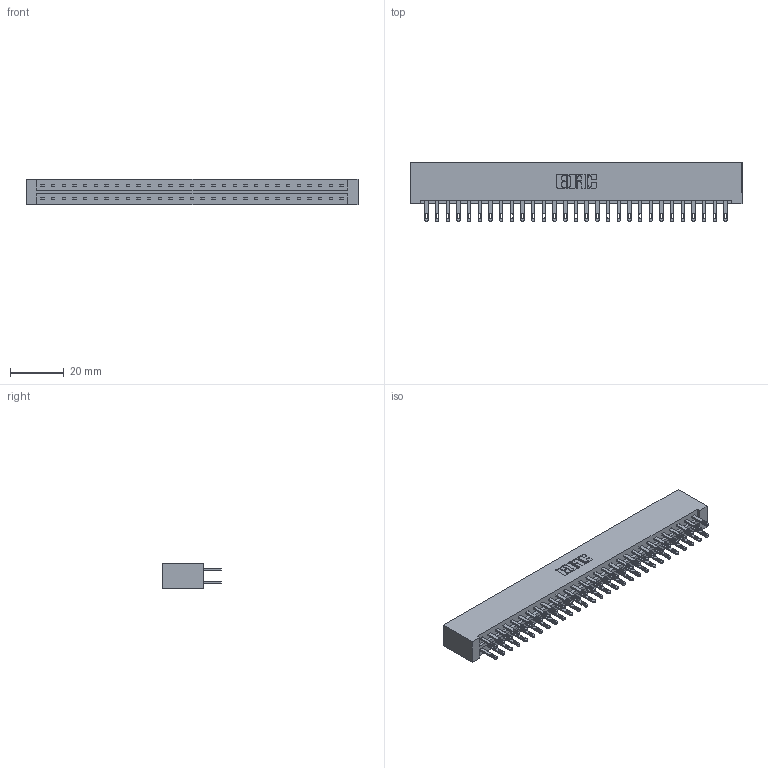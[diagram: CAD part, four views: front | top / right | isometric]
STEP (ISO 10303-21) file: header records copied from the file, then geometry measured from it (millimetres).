
FILE_DESCRIPTION (( 'STEP AP203' ), '1' );
FILE_NAME ('833-058-500-201.STEP', '2020-06-04T23:47:11', ( '' ), ( '' ), 'SwSTEP 2.0', 'SolidWorks 2020', '' );
FILE_SCHEMA (( 'CONFIG_CONTROL_DESIGN' ));
Length unit declared in the file: inch
Products named in the file (3): 345-292-001_345-293-100; 833-058-500-201; 833 Part_Lugless
Assembly tree (59 placements, depth 2):
  833-058-500-201
    833 Part_Lugless
    345-292-001_345-293-100  x58
Bounding box: 123.16 x 21.85 x 9.4 mm (x, y, z)
Volume: 13262.3 mm3; surface area: 16202.3 mm2
Topology: 59 solids, 59 shells, 2890 faces, 8813 edges, 5874 vertices
Faces by surface type: plane 1806, cylinder 1084
Entity records: 19991 total; most frequent: CARTESIAN_POINT 3326, ORIENTED_EDGE 3262, DIRECTION 2859, EDGE_CURVE 1631, LINE 1507, VECTOR 1507, VERTEX_POINT 1086, AXIS2_PLACEMENT_3D 676
